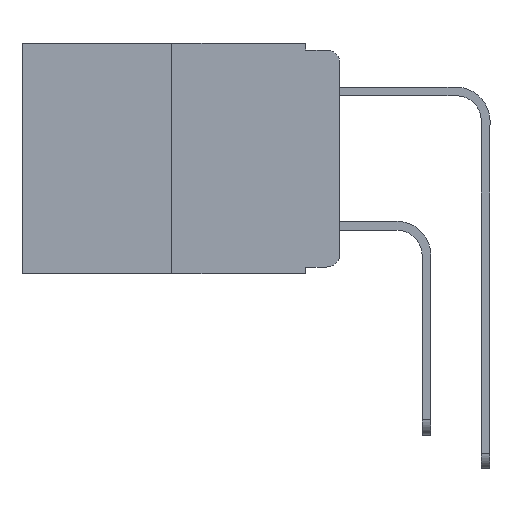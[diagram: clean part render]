
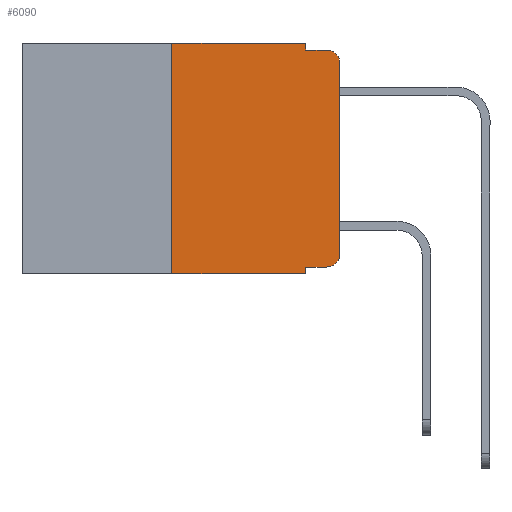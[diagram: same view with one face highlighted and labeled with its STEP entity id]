
A CAD part, left-side view. The second image highlights one B-rep face of the part: STEP entity #6090.
In plain terms, the highlighted planar face has unit normal (-1, 0, 0).
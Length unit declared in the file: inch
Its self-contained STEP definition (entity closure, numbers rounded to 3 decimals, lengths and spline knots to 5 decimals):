
#189 = CARTESIAN_POINT ( 'NONE',  ( 0., 0.02, -0.03 ) ) ;
#370 = DIRECTION ( 'NONE',  ( 0., -1., 0. ) ) ;
#410 = ORIENTED_EDGE ( 'NONE', *, *, #14075, .T. ) ;
#431 = ORIENTED_EDGE ( 'NONE', *, *, #14715, .T. ) ;
#605 = ORIENTED_EDGE ( 'NONE', *, *, #5194, .F. ) ;
#795 = EDGE_CURVE ( 'NONE', #6155, #8454, #13537, .T. ) ;
#973 = EDGE_CURVE ( 'NONE', #4930, #3856, #4906, .T. ) ;
#1128 = CARTESIAN_POINT ( 'NONE',  ( 0., 0.25, -0.343 ) ) ;
#1155 = VECTOR ( 'NONE', #13825, 39.37008 ) ;
#1284 = VECTOR ( 'NONE', #11993, 39.37008 ) ;
#1352 = ORIENTED_EDGE ( 'NONE', *, *, #973, .F. ) ;
#1371 = CARTESIAN_POINT ( 'NONE',  ( 0., 0.051, -0.333 ) ) ;
#1419 = ORIENTED_EDGE ( 'NONE', *, *, #11615, .T. ) ;
#1444 = DIRECTION ( 'NONE',  ( 0., 0., -1. ) ) ;
#1474 = VECTOR ( 'NONE', #7132, 39.37008 ) ;
#1514 = VECTOR ( 'NONE', #11310, 39.37008 ) ;
#1713 = EDGE_CURVE ( 'NONE', #6155, #6287, #10537, .T. ) ;
#1961 = LINE ( 'NONE', #5179, #13907 ) ;
#1988 = AXIS2_PLACEMENT_3D ( 'NONE', #189, #8536, #1444 ) ;
#2485 = DIRECTION ( 'NONE',  ( 0., 0., -1. ) ) ;
#2969 = DIRECTION ( 'NONE',  ( -1., 0., 0. ) ) ;
#3421 = ORIENTED_EDGE ( 'NONE', *, *, #795, .T. ) ;
#3430 = CARTESIAN_POINT ( 'NONE',  ( 0., 0.051, -0.01 ) ) ;
#3593 = ORIENTED_EDGE ( 'NONE', *, *, #1713, .F. ) ;
#3626 = PLANE ( 'NONE',  #7484 ) ;
#3750 = EDGE_CURVE ( 'NONE', #3856, #9585, #10871, .T. ) ;
#3856 = VERTEX_POINT ( 'NONE', #9552 ) ;
#4187 = VERTEX_POINT ( 'NONE', #14803 ) ;
#4310 = ORIENTED_EDGE ( 'NONE', *, *, #3750, .F. ) ;
#4906 = LINE ( 'NONE', #10387, #5290 ) ;
#4930 = VERTEX_POINT ( 'NONE', #1128 ) ;
#5057 = CARTESIAN_POINT ( 'NONE',  ( 0., 0.473, -0.343 ) ) ;
#5099 = EDGE_CURVE ( 'NONE', #9585, #8723, #12156, .T. ) ;
#5137 = CIRCLE ( 'NONE', #1988, 0.02 ) ;
#5148 = CARTESIAN_POINT ( 'NONE',  ( 0., 0.051, -0.343 ) ) ;
#5179 = CARTESIAN_POINT ( 'NONE',  ( 0., 0.051, -0.01 ) ) ;
#5194 = EDGE_CURVE ( 'NONE', #8723, #4187, #1961, .T. ) ;
#5288 = ORIENTED_EDGE ( 'NONE', *, *, #5099, .F. ) ;
#5290 = VECTOR ( 'NONE', #10973, 39.37008 ) ;
#5474 = VERTEX_POINT ( 'NONE', #5742 ) ;
#5742 = CARTESIAN_POINT ( 'NONE',  ( 0., 0., -0.313 ) ) ;
#6090 = ADVANCED_FACE ( 'NONE', ( #14896 ), #3626, .F. ) ;
#6136 = CARTESIAN_POINT ( 'NONE',  ( 0., 0., 0. ) ) ;
#6141 = CIRCLE ( 'NONE', #14065, 0.02 ) ;
#6155 = VERTEX_POINT ( 'NONE', #1371 ) ;
#6287 = VERTEX_POINT ( 'NONE', #5148 ) ;
#6429 = VECTOR ( 'NONE', #8549, 39.37008 ) ;
#6802 = ORIENTED_EDGE ( 'NONE', *, *, #13203, .T. ) ;
#7012 = CARTESIAN_POINT ( 'NONE',  ( 0., 0.051, -0.333 ) ) ;
#7132 = DIRECTION ( 'NONE',  ( 0., -1., 0. ) ) ;
#7417 = CARTESIAN_POINT ( 'NONE',  ( 0., 0.051, 0. ) ) ;
#7484 = AXIS2_PLACEMENT_3D ( 'NONE', #8377, #9548, #2485 ) ;
#7919 = CARTESIAN_POINT ( 'NONE',  ( 0., 0., -0.03 ) ) ;
#8377 = CARTESIAN_POINT ( 'NONE',  ( 0., 0.473, 0. ) ) ;
#8454 = VERTEX_POINT ( 'NONE', #8868 ) ;
#8536 = DIRECTION ( 'NONE',  ( -1., 0., 0. ) ) ;
#8549 = DIRECTION ( 'NONE',  ( 0., 0., -1. ) ) ;
#8723 = VERTEX_POINT ( 'NONE', #3430 ) ;
#8868 = CARTESIAN_POINT ( 'NONE',  ( 0., 0.02, -0.333 ) ) ;
#9192 = VECTOR ( 'NONE', #12871, 39.37008 ) ;
#9548 = DIRECTION ( 'NONE',  ( 1., 0., 0. ) ) ;
#9552 = CARTESIAN_POINT ( 'NONE',  ( 0., 0.25, 0. ) ) ;
#9585 = VERTEX_POINT ( 'NONE', #14263 ) ;
#9998 = CARTESIAN_POINT ( 'NONE',  ( 0., 0.02, -0.313 ) ) ;
#10162 = CARTESIAN_POINT ( 'NONE',  ( 0., 0.051, 0. ) ) ;
#10387 = CARTESIAN_POINT ( 'NONE',  ( 0., 0.25, 0. ) ) ;
#10537 = LINE ( 'NONE', #10162, #1514 ) ;
#10685 = LINE ( 'NONE', #5057, #1284 ) ;
#10871 = LINE ( 'NONE', #12793, #1474 ) ;
#10973 = DIRECTION ( 'NONE',  ( 0., 0., 1. ) ) ;
#11155 = DIRECTION ( 'NONE',  ( 0., 0., -1. ) ) ;
#11267 = EDGE_LOOP ( 'NONE', ( #410, #431, #605, #5288, #4310, #1352, #1419, #3593, #3421, #6802 ) ) ;
#11298 = VERTEX_POINT ( 'NONE', #7919 ) ;
#11310 = DIRECTION ( 'NONE',  ( 0., 0., -1. ) ) ;
#11615 = EDGE_CURVE ( 'NONE', #4930, #6287, #10685, .T. ) ;
#11993 = DIRECTION ( 'NONE',  ( 0., -1., 0. ) ) ;
#12156 = LINE ( 'NONE', #7417, #6429 ) ;
#12793 = CARTESIAN_POINT ( 'NONE',  ( 0., 0.473, 0. ) ) ;
#12871 = DIRECTION ( 'NONE',  ( 0., 0., 1. ) ) ;
#13203 = EDGE_CURVE ( 'NONE', #8454, #5474, #6141, .T. ) ;
#13537 = LINE ( 'NONE', #7012, #1155 ) ;
#13825 = DIRECTION ( 'NONE',  ( 0., -1., 0. ) ) ;
#13907 = VECTOR ( 'NONE', #370, 39.37008 ) ;
#14065 = AXIS2_PLACEMENT_3D ( 'NONE', #9998, #2969, #11155 ) ;
#14075 = EDGE_CURVE ( 'NONE', #5474, #11298, #14777, .T. ) ;
#14263 = CARTESIAN_POINT ( 'NONE',  ( 0., 0.051, 0. ) ) ;
#14715 = EDGE_CURVE ( 'NONE', #11298, #4187, #5137, .T. ) ;
#14777 = LINE ( 'NONE', #6136, #9192 ) ;
#14803 = CARTESIAN_POINT ( 'NONE',  ( 0., 0.02, -0.01 ) ) ;
#14896 = FACE_OUTER_BOUND ( 'NONE', #11267, .T. ) ;
